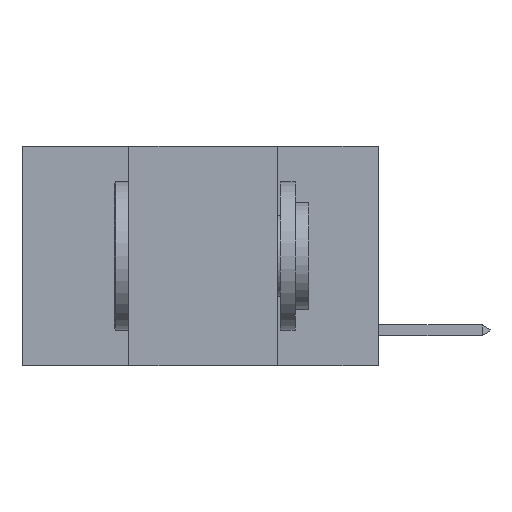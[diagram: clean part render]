
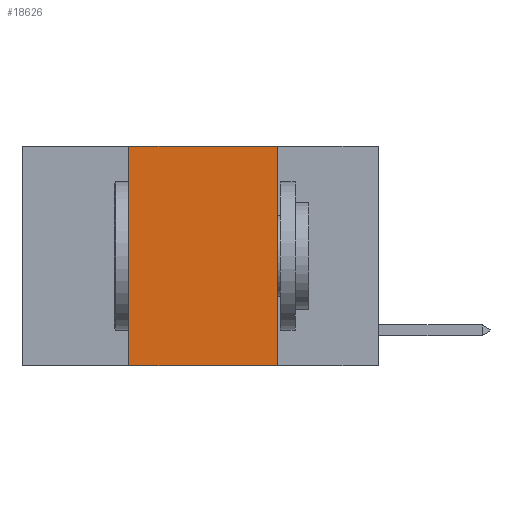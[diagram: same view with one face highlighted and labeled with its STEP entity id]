
A CAD part, left-side view. The second image highlights one B-rep face of the part: STEP entity #18626.
In plain terms, the highlighted planar face has unit normal (-1, 0, 0).
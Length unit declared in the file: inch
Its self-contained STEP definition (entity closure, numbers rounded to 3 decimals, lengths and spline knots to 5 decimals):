
#84 = CARTESIAN_POINT ( 'NONE',  ( 0., 0.6, 0. ) ) ;
#89 = EDGE_CURVE ( 'NONE', #13389, #2987, #3430, .T. ) ;
#305 = VECTOR ( 'NONE', #3589, 39.37008 ) ;
#1040 = CARTESIAN_POINT ( 'NONE',  ( 0., 0.42, -0.37 ) ) ;
#1087 = ORIENTED_EDGE ( 'NONE', *, *, #89, .T. ) ;
#2694 = ORIENTED_EDGE ( 'NONE', *, *, #3930, .F. ) ;
#2987 = VERTEX_POINT ( 'NONE', #19360 ) ;
#3430 = LINE ( 'NONE', #21734, #9039 ) ;
#3589 = DIRECTION ( 'NONE',  ( 0., 0., 1. ) ) ;
#3693 = CARTESIAN_POINT ( 'NONE',  ( 0., 0.42, 0. ) ) ;
#3930 = EDGE_CURVE ( 'NONE', #13389, #6203, #5395, .T. ) ;
#4066 = CARTESIAN_POINT ( 'NONE',  ( 0., 0.42, 0. ) ) ;
#5395 = LINE ( 'NONE', #3693, #305 ) ;
#5790 = ORIENTED_EDGE ( 'NONE', *, *, #13003, .F. ) ;
#6203 = VERTEX_POINT ( 'NONE', #4066 ) ;
#7326 = CARTESIAN_POINT ( 'NONE',  ( 0., 0.17, 0. ) ) ;
#8590 = EDGE_LOOP ( 'NONE', ( #9061, #5790, #2694, #1087 ) ) ;
#8998 = EDGE_CURVE ( 'NONE', #16998, #2987, #20129, .T. ) ;
#9039 = VECTOR ( 'NONE', #21703, 39.37008 ) ;
#9061 = ORIENTED_EDGE ( 'NONE', *, *, #8998, .F. ) ;
#9149 = DIRECTION ( 'NONE',  ( 1., 0., 0. ) ) ;
#10351 = VECTOR ( 'NONE', #18413, 39.37008 ) ;
#11525 = DIRECTION ( 'NONE',  ( 0., -1., 0. ) ) ;
#12406 = FACE_OUTER_BOUND ( 'NONE', #8590, .T. ) ;
#13003 = EDGE_CURVE ( 'NONE', #6203, #16998, #19100, .T. ) ;
#13389 = VERTEX_POINT ( 'NONE', #1040 ) ;
#13695 = CARTESIAN_POINT ( 'NONE',  ( 0., 0.17, 0. ) ) ;
#14218 = VECTOR ( 'NONE', #11525, 39.37008 ) ;
#16519 = PLANE ( 'NONE',  #17271 ) ;
#16998 = VERTEX_POINT ( 'NONE', #13695 ) ;
#17271 = AXIS2_PLACEMENT_3D ( 'NONE', #20201, #9149, #22035 ) ;
#18413 = DIRECTION ( 'NONE',  ( 0., 0., -1. ) ) ;
#18626 = ADVANCED_FACE ( 'NONE', ( #12406 ), #16519, .F. ) ;
#19100 = LINE ( 'NONE', #84, #14218 ) ;
#19360 = CARTESIAN_POINT ( 'NONE',  ( 0., 0.17, -0.37 ) ) ;
#20129 = LINE ( 'NONE', #7326, #10351 ) ;
#20201 = CARTESIAN_POINT ( 'NONE',  ( 0., 0.6, 0. ) ) ;
#21703 = DIRECTION ( 'NONE',  ( 0., -1., 0. ) ) ;
#21734 = CARTESIAN_POINT ( 'NONE',  ( 0., 0.6, -0.37 ) ) ;
#22035 = DIRECTION ( 'NONE',  ( 0., 0., -1. ) ) ;
